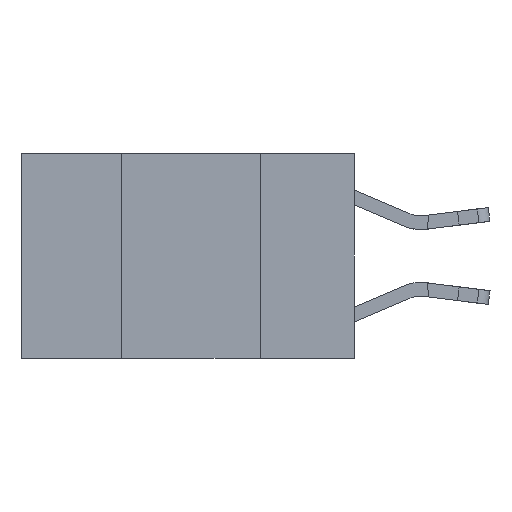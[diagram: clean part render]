
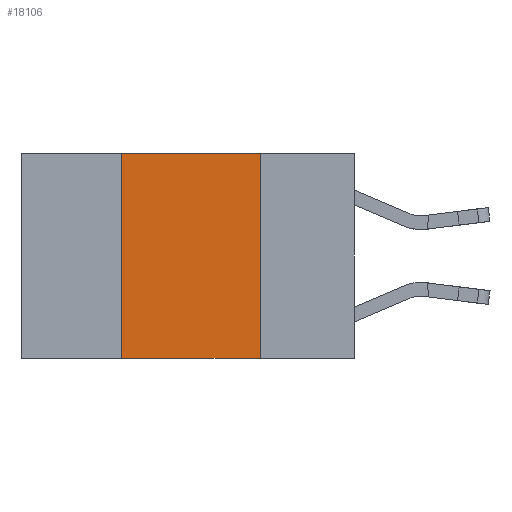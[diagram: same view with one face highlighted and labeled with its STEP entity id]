
A CAD part, left-side view. The second image highlights one B-rep face of the part: STEP entity #18106.
In plain terms, the highlighted planar face has unit normal (-1, 0, 0).
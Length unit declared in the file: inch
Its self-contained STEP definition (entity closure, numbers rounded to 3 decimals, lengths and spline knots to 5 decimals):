
#338 = LINE ( 'NONE', #7217, #18006 ) ;
#429 = EDGE_LOOP ( 'NONE', ( #19052, #13248, #7329, #14635 ) ) ;
#852 = CARTESIAN_POINT ( 'NONE',  ( 0., 0.42, 0. ) ) ;
#1777 = DIRECTION ( 'NONE',  ( 0., 0., 1. ) ) ;
#2891 = EDGE_CURVE ( 'NONE', #18658, #14729, #22148, .T. ) ;
#3827 = VERTEX_POINT ( 'NONE', #852 ) ;
#4345 = LINE ( 'NONE', #14490, #5673 ) ;
#4893 = EDGE_CURVE ( 'NONE', #12326, #14729, #17683, .T. ) ;
#5673 = VECTOR ( 'NONE', #1777, 39.37008 ) ;
#6371 = CARTESIAN_POINT ( 'NONE',  ( 0., 0.6, -0.37 ) ) ;
#7217 = CARTESIAN_POINT ( 'NONE',  ( 0., 0.6, 0. ) ) ;
#7329 = ORIENTED_EDGE ( 'NONE', *, *, #12154, .F. ) ;
#8533 = DIRECTION ( 'NONE',  ( 0., -1., 0. ) ) ;
#8545 = PLANE ( 'NONE',  #18048 ) ;
#10698 = DIRECTION ( 'NONE',  ( 0., 0., -1. ) ) ;
#11734 = FACE_OUTER_BOUND ( 'NONE', #429, .T. ) ;
#12154 = EDGE_CURVE ( 'NONE', #18658, #3827, #4345, .T. ) ;
#12326 = VERTEX_POINT ( 'NONE', #23526 ) ;
#13248 = ORIENTED_EDGE ( 'NONE', *, *, #22525, .F. ) ;
#13627 = DIRECTION ( 'NONE',  ( 0., -1., 0. ) ) ;
#14172 = DIRECTION ( 'NONE',  ( 0., 0., -1. ) ) ;
#14467 = CARTESIAN_POINT ( 'NONE',  ( 0., 0.42, -0.37 ) ) ;
#14490 = CARTESIAN_POINT ( 'NONE',  ( 0., 0.42, 0. ) ) ;
#14635 = ORIENTED_EDGE ( 'NONE', *, *, #2891, .T. ) ;
#14729 = VERTEX_POINT ( 'NONE', #15713 ) ;
#15713 = CARTESIAN_POINT ( 'NONE',  ( 0., 0.17, -0.37 ) ) ;
#17683 = LINE ( 'NONE', #24813, #22700 ) ;
#18006 = VECTOR ( 'NONE', #13627, 39.37008 ) ;
#18048 = AXIS2_PLACEMENT_3D ( 'NONE', #19176, #23447, #10698 ) ;
#18106 = ADVANCED_FACE ( 'NONE', ( #11734 ), #8545, .F. ) ;
#18658 = VERTEX_POINT ( 'NONE', #14467 ) ;
#19052 = ORIENTED_EDGE ( 'NONE', *, *, #4893, .F. ) ;
#19176 = CARTESIAN_POINT ( 'NONE',  ( 0., 0.6, 0. ) ) ;
#22148 = LINE ( 'NONE', #6371, #22830 ) ;
#22525 = EDGE_CURVE ( 'NONE', #3827, #12326, #338, .T. ) ;
#22700 = VECTOR ( 'NONE', #14172, 39.37008 ) ;
#22830 = VECTOR ( 'NONE', #8533, 39.37008 ) ;
#23447 = DIRECTION ( 'NONE',  ( 1., 0., 0. ) ) ;
#23526 = CARTESIAN_POINT ( 'NONE',  ( 0., 0.17, 0. ) ) ;
#24813 = CARTESIAN_POINT ( 'NONE',  ( 0., 0.17, 0. ) ) ;
